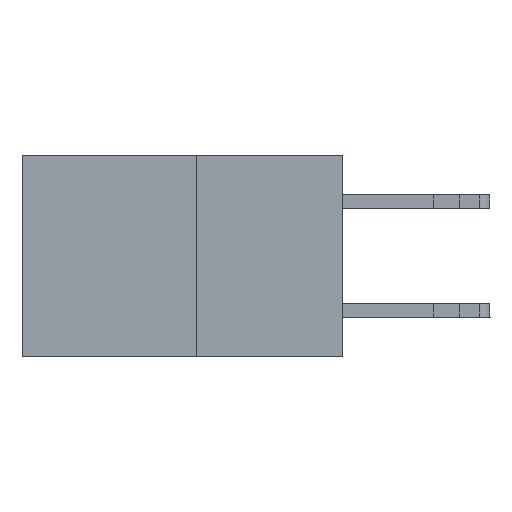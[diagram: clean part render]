
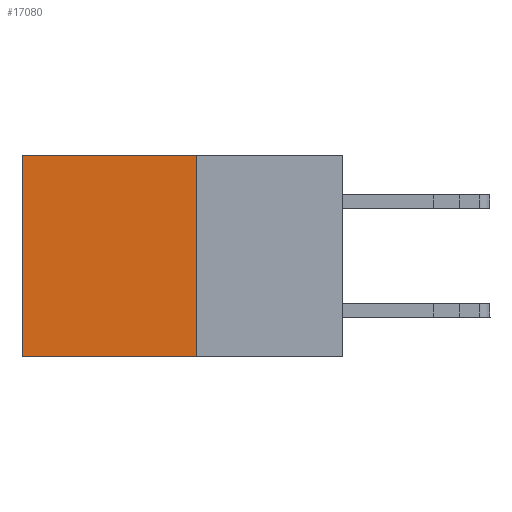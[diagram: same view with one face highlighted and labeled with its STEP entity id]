
A CAD part, left-side view. The second image highlights one B-rep face of the part: STEP entity #17080.
In plain terms, the highlighted planar face has unit normal (-1, 0, 0).
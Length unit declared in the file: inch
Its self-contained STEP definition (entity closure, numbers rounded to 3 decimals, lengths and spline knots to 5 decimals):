
#889 = VERTEX_POINT ( 'NONE', #10406 ) ;
#1550 = LINE ( 'NONE', #20422, #5423 ) ;
#2456 = EDGE_CURVE ( 'NONE', #889, #10255, #15367, .T. ) ;
#3271 = DIRECTION ( 'NONE',  ( 0., 0., -1. ) ) ;
#4288 = AXIS2_PLACEMENT_3D ( 'NONE', #11374, #4748, #16326 ) ;
#4748 = DIRECTION ( 'NONE',  ( 1., 0., 0. ) ) ;
#5423 = VECTOR ( 'NONE', #18909, 39.37008 ) ;
#5589 = VERTEX_POINT ( 'NONE', #7046 ) ;
#5753 = DIRECTION ( 'NONE',  ( 0., 1., 0. ) ) ;
#6952 = ORIENTED_EDGE ( 'NONE', *, *, #8955, .T. ) ;
#7046 = CARTESIAN_POINT ( 'NONE',  ( 0.277, 0.59, 0. ) ) ;
#7748 = EDGE_LOOP ( 'NONE', ( #6952, #8239, #16315, #17905 ) ) ;
#8202 = CARTESIAN_POINT ( 'NONE',  ( 0.277, 0.59, -0.37 ) ) ;
#8239 = ORIENTED_EDGE ( 'NONE', *, *, #13886, .F. ) ;
#8955 = EDGE_CURVE ( 'NONE', #5589, #14132, #14715, .T. ) ;
#9174 = VECTOR ( 'NONE', #5753, 39.37008 ) ;
#9667 = CARTESIAN_POINT ( 'NONE',  ( 0.277, 0.59, -0.37 ) ) ;
#10255 = VERTEX_POINT ( 'NONE', #17718 ) ;
#10263 = VECTOR ( 'NONE', #3271, 39.37008 ) ;
#10406 = CARTESIAN_POINT ( 'NONE',  ( 0.277, 0.27, 0. ) ) ;
#11374 = CARTESIAN_POINT ( 'NONE',  ( 0.277, 0.27, -0.37 ) ) ;
#11421 = FACE_OUTER_BOUND ( 'NONE', #7748, .T. ) ;
#13886 = EDGE_CURVE ( 'NONE', #10255, #14132, #17429, .T. ) ;
#14062 = CARTESIAN_POINT ( 'NONE',  ( 0.277, 0.27, -0.37 ) ) ;
#14132 = VERTEX_POINT ( 'NONE', #9667 ) ;
#14715 = LINE ( 'NONE', #8202, #10263 ) ;
#15367 = LINE ( 'NONE', #19275, #17626 ) ;
#16315 = ORIENTED_EDGE ( 'NONE', *, *, #2456, .F. ) ;
#16326 = DIRECTION ( 'NONE',  ( 0., 0., -1. ) ) ;
#17080 = ADVANCED_FACE ( 'NONE', ( #11421 ), #17884, .F. ) ;
#17355 = EDGE_CURVE ( 'NONE', #889, #5589, #1550, .T. ) ;
#17429 = LINE ( 'NONE', #14062, #9174 ) ;
#17626 = VECTOR ( 'NONE', #19144, 39.37008 ) ;
#17718 = CARTESIAN_POINT ( 'NONE',  ( 0.277, 0.27, -0.37 ) ) ;
#17884 = PLANE ( 'NONE',  #4288 ) ;
#17905 = ORIENTED_EDGE ( 'NONE', *, *, #17355, .T. ) ;
#18909 = DIRECTION ( 'NONE',  ( 0., 1., 0. ) ) ;
#19144 = DIRECTION ( 'NONE',  ( 0., 0., -1. ) ) ;
#19275 = CARTESIAN_POINT ( 'NONE',  ( 0.277, 0.27, -0.37 ) ) ;
#20422 = CARTESIAN_POINT ( 'NONE',  ( 0.277, 0.27, 0. ) ) ;
